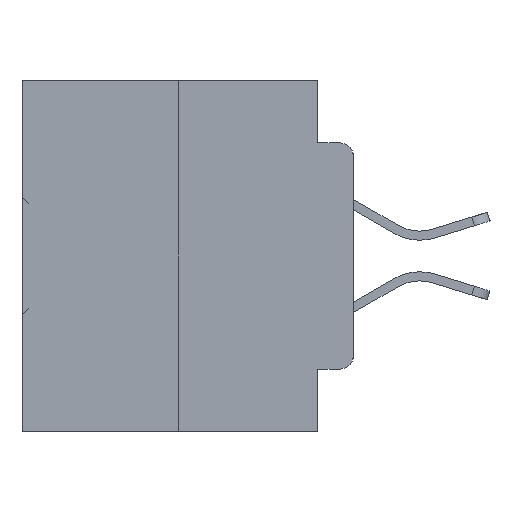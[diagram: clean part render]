
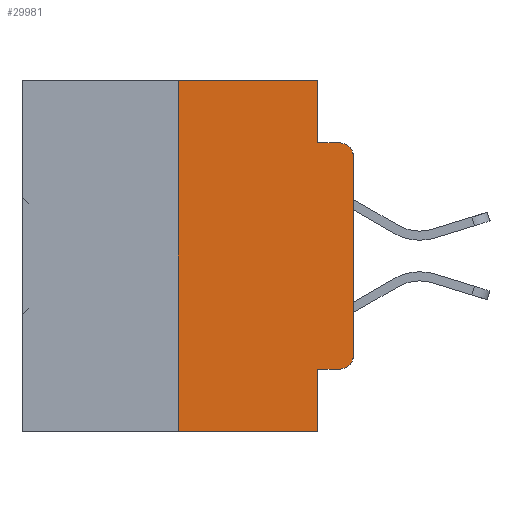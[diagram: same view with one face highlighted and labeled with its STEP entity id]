
A CAD part, left-side view. The second image highlights one B-rep face of the part: STEP entity #29981.
In plain terms, the highlighted planar face has unit normal (-1, 0, 0).
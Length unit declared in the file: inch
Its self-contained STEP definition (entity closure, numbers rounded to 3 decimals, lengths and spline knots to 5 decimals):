
#87 = VERTEX_POINT ( 'NONE', #25305 ) ;
#329 = LINE ( 'NONE', #35622, #36534 ) ;
#453 = VERTEX_POINT ( 'NONE', #28134 ) ;
#521 = DIRECTION ( 'NONE',  ( 0., 0., 1. ) ) ;
#1131 = VERTEX_POINT ( 'NONE', #33052 ) ;
#2206 = ORIENTED_EDGE ( 'NONE', *, *, #34347, .F. ) ;
#2283 = ORIENTED_EDGE ( 'NONE', *, *, #37071, .T. ) ;
#3017 = VERTEX_POINT ( 'NONE', #30692 ) ;
#3918 = CARTESIAN_POINT ( 'NONE',  ( 0., 0.051, 0. ) ) ;
#6854 = CARTESIAN_POINT ( 'NONE',  ( 0., 0.051, -0.4115 ) ) ;
#8697 = LINE ( 'NONE', #26164, #21003 ) ;
#8931 = EDGE_CURVE ( 'NONE', #3017, #26769, #18445, .T. ) ;
#8991 = DIRECTION ( 'NONE',  ( 1., 0., 0. ) ) ;
#9567 = ORIENTED_EDGE ( 'NONE', *, *, #8931, .T. ) ;
#9678 = VERTEX_POINT ( 'NONE', #6854 ) ;
#9794 = VECTOR ( 'NONE', #29971, 39.37008 ) ;
#9807 = ORIENTED_EDGE ( 'NONE', *, *, #17945, .F. ) ;
#9893 = VECTOR ( 'NONE', #19852, 39.37008 ) ;
#10047 = VERTEX_POINT ( 'NONE', #25166 ) ;
#10125 = VECTOR ( 'NONE', #27618, 39.37008 ) ;
#10246 = VECTOR ( 'NONE', #19022, 39.37008 ) ;
#10557 = EDGE_CURVE ( 'NONE', #453, #87, #13581, .T. ) ;
#11316 = PLANE ( 'NONE',  #16425 ) ;
#11708 = EDGE_CURVE ( 'NONE', #18122, #10047, #16931, .T. ) ;
#11744 = EDGE_CURVE ( 'NONE', #10047, #3017, #329, .T. ) ;
#12029 = CARTESIAN_POINT ( 'NONE',  ( 0., 0.02, -0.3915 ) ) ;
#12489 = VECTOR ( 'NONE', #26773, 39.37008 ) ;
#13581 = LINE ( 'NONE', #36991, #10125 ) ;
#13801 = EDGE_CURVE ( 'NONE', #28735, #1131, #8697, .T. ) ;
#13912 = CARTESIAN_POINT ( 'NONE',  ( 0., 0.25, 0. ) ) ;
#14763 = EDGE_CURVE ( 'NONE', #30082, #26769, #17941, .T. ) ;
#15485 = DIRECTION ( 'NONE',  ( 0., 0., -1. ) ) ;
#15630 = DIRECTION ( 'NONE',  ( 0., 0., -1. ) ) ;
#16425 = AXIS2_PLACEMENT_3D ( 'NONE', #23185, #8991, #37773 ) ;
#16651 = ORIENTED_EDGE ( 'NONE', *, *, #13801, .F. ) ;
#16738 = ORIENTED_EDGE ( 'NONE', *, *, #11708, .T. ) ;
#16931 = CIRCLE ( 'NONE', #26742, 0.02 ) ;
#17082 = ORIENTED_EDGE ( 'NONE', *, *, #14763, .F. ) ;
#17445 = DIRECTION ( 'NONE',  ( -1., 0., 0. ) ) ;
#17538 = CARTESIAN_POINT ( 'NONE',  ( 0., 0.02, -0.4115 ) ) ;
#17941 = LINE ( 'NONE', #32718, #12489 ) ;
#17945 = EDGE_CURVE ( 'NONE', #453, #28735, #25631, .T. ) ;
#18122 = VERTEX_POINT ( 'NONE', #17538 ) ;
#18445 = CIRCLE ( 'NONE', #28240, 0.02 ) ;
#19022 = DIRECTION ( 'NONE',  ( 0., 0., -1. ) ) ;
#19852 = DIRECTION ( 'NONE',  ( 0., 0., 1. ) ) ;
#19875 = ORIENTED_EDGE ( 'NONE', *, *, #10557, .T. ) ;
#19944 = DIRECTION ( 'NONE',  ( 0., 0., -1. ) ) ;
#20073 = VECTOR ( 'NONE', #15630, 39.37008 ) ;
#20493 = EDGE_LOOP ( 'NONE', ( #21854, #9567, #17082, #2206, #16651, #9807, #19875, #34349, #2283, #16738 ) ) ;
#21003 = VECTOR ( 'NONE', #34216, 39.37008 ) ;
#21234 = DIRECTION ( 'NONE',  ( -1., 0., 0. ) ) ;
#21854 = ORIENTED_EDGE ( 'NONE', *, *, #11744, .T. ) ;
#21901 = CARTESIAN_POINT ( 'NONE',  ( 0., 0.051, 0. ) ) ;
#23185 = CARTESIAN_POINT ( 'NONE',  ( 0., 0.473, 0. ) ) ;
#25166 = CARTESIAN_POINT ( 'NONE',  ( 0., 0., -0.3915 ) ) ;
#25305 = CARTESIAN_POINT ( 'NONE',  ( 0., 0.051, -0.5 ) ) ;
#25631 = LINE ( 'NONE', #13912, #9893 ) ;
#26164 = CARTESIAN_POINT ( 'NONE',  ( 0., 0.473, 0. ) ) ;
#26742 = AXIS2_PLACEMENT_3D ( 'NONE', #12029, #21234, #15485 ) ;
#26769 = VERTEX_POINT ( 'NONE', #35580 ) ;
#26773 = DIRECTION ( 'NONE',  ( 0., -1., 0. ) ) ;
#26953 = EDGE_CURVE ( 'NONE', #9678, #87, #30206, .T. ) ;
#27618 = DIRECTION ( 'NONE',  ( 0., -1., 0. ) ) ;
#28134 = CARTESIAN_POINT ( 'NONE',  ( 0., 0.25, -0.5 ) ) ;
#28240 = AXIS2_PLACEMENT_3D ( 'NONE', #34545, #17445, #19944 ) ;
#28735 = VERTEX_POINT ( 'NONE', #33855 ) ;
#29214 = LINE ( 'NONE', #32276, #9794 ) ;
#29971 = DIRECTION ( 'NONE',  ( 0., -1., 0. ) ) ;
#29981 = ADVANCED_FACE ( 'NONE', ( #32396 ), #11316, .F. ) ;
#30082 = VERTEX_POINT ( 'NONE', #35841 ) ;
#30206 = LINE ( 'NONE', #3918, #20073 ) ;
#30692 = CARTESIAN_POINT ( 'NONE',  ( 0., 0., -0.1085 ) ) ;
#32276 = CARTESIAN_POINT ( 'NONE',  ( 0., 0.051, -0.4115 ) ) ;
#32396 = FACE_OUTER_BOUND ( 'NONE', #20493, .T. ) ;
#32718 = CARTESIAN_POINT ( 'NONE',  ( 0., 0.051, -0.0885 ) ) ;
#33052 = CARTESIAN_POINT ( 'NONE',  ( 0., 0.051, 0. ) ) ;
#33855 = CARTESIAN_POINT ( 'NONE',  ( 0., 0.25, 0. ) ) ;
#34164 = LINE ( 'NONE', #21901, #10246 ) ;
#34216 = DIRECTION ( 'NONE',  ( 0., -1., 0. ) ) ;
#34347 = EDGE_CURVE ( 'NONE', #1131, #30082, #34164, .T. ) ;
#34349 = ORIENTED_EDGE ( 'NONE', *, *, #26953, .F. ) ;
#34545 = CARTESIAN_POINT ( 'NONE',  ( 0., 0.02, -0.1085 ) ) ;
#35580 = CARTESIAN_POINT ( 'NONE',  ( 0., 0.02, -0.0885 ) ) ;
#35622 = CARTESIAN_POINT ( 'NONE',  ( 0., 0., 0. ) ) ;
#35841 = CARTESIAN_POINT ( 'NONE',  ( 0., 0.051, -0.0885 ) ) ;
#36534 = VECTOR ( 'NONE', #521, 39.37008 ) ;
#36991 = CARTESIAN_POINT ( 'NONE',  ( 0., 0.473, -0.5 ) ) ;
#37071 = EDGE_CURVE ( 'NONE', #9678, #18122, #29214, .T. ) ;
#37773 = DIRECTION ( 'NONE',  ( 0., 0., -1. ) ) ;
